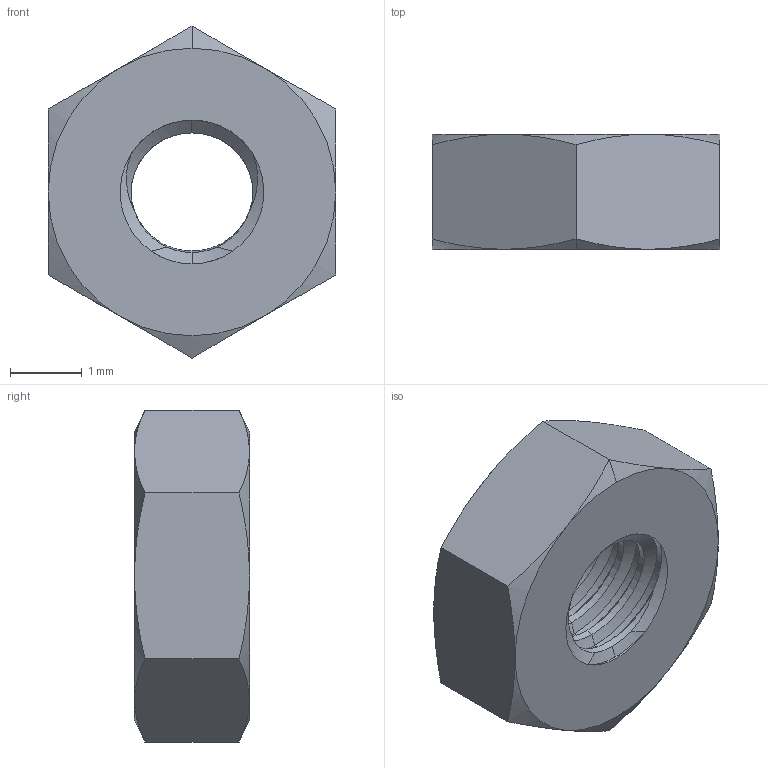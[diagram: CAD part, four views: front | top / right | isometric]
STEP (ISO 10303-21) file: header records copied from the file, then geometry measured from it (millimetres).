
FILE_DESCRIPTION (( 'STEP AP214' ), '1' );
FILE_NAME ('Hinge_Nut_90592A004.step', '2013-11-06T14:31:11', ( 'elpi' ), ( '' ), 'SwSTEP 2.0', 'SolidWorks 2013', '' );
FILE_SCHEMA (( 'AUTOMOTIVE_DESIGN' ));
Length unit declared in the file: millimetre
Products named in the file (1): Hinge_Nut_90592A004
Bounding box: 4 x 1.6 x 4.62 mm (x, y, z)
Volume: 17.8 mm3; surface area: 56.3 mm2
Topology: 1 solids, 1 shells, 64 faces, 139 edges, 77 vertices
Faces by surface type: cone 36, cylinder 20, plane 8
Entity records: 1993 total; most frequent: CARTESIAN_POINT 661, ORIENTED_EDGE 278, DIRECTION 255, EDGE_CURVE 139, AXIS2_PLACEMENT_3D 109, VERTEX_POINT 77, EDGE_LOOP 66, FACE_OUTER_BOUND 64
